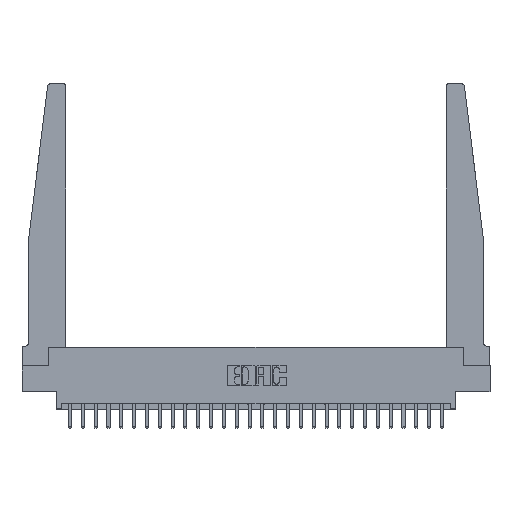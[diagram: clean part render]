
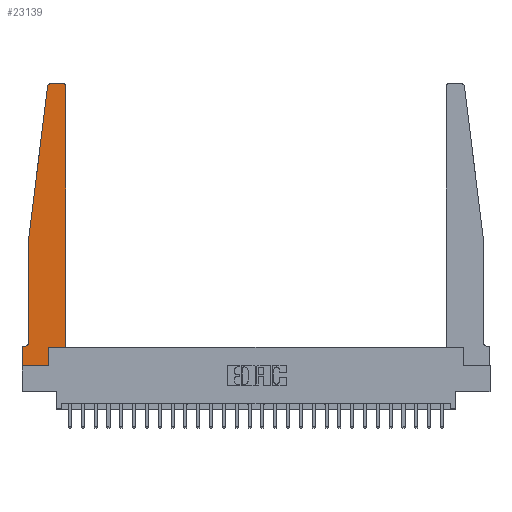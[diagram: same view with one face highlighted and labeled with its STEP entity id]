
A CAD part, top view. The second image highlights one B-rep face of the part: STEP entity #23139.
In plain terms, the highlighted planar face has unit normal (0, 0, 1).
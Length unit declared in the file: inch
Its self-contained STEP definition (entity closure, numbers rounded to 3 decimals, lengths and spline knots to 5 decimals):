
#36 = ORIENTED_EDGE ( 'NONE', *, *, #348, .T. ) ;
#49 = LINE ( 'NONE', #11934, #21082 ) ;
#164 = DIRECTION ( 'NONE',  ( -1., 0., 0. ) ) ;
#248 = CARTESIAN_POINT ( 'NONE',  ( 0., 0.1875, 0.37 ) ) ;
#348 = EDGE_CURVE ( 'NONE', #454, #18838, #3768, .T. ) ;
#454 = VERTEX_POINT ( 'NONE', #20134 ) ;
#847 = AXIS2_PLACEMENT_3D ( 'NONE', #1328, #15549, #3390 ) ;
#1015 = VECTOR ( 'NONE', #18648, 39.37008 ) ;
#1196 = CARTESIAN_POINT ( 'NONE',  ( 0.2605, 0.18, 0.37 ) ) ;
#1328 = CARTESIAN_POINT ( 'NONE',  ( 0.27653, 2.72, 0.37 ) ) ;
#1387 = CIRCLE ( 'NONE', #7462, 0.03 ) ;
#1421 = VECTOR ( 'NONE', #20547, 39.37008 ) ;
#1506 = DIRECTION ( 'NONE',  ( 1., 0., 0. ) ) ;
#1509 = DIRECTION ( 'NONE',  ( 0., 0., 1. ) ) ;
#1545 = CARTESIAN_POINT ( 'NONE',  ( 0.395, 2.72, 0.37 ) ) ;
#1833 = VECTOR ( 'NONE', #23311, 39.37008 ) ;
#2065 = ORIENTED_EDGE ( 'NONE', *, *, #13735, .T. ) ;
#2157 = VECTOR ( 'NONE', #19531, 39.37008 ) ;
#2487 = LINE ( 'NONE', #17197, #1833 ) ;
#2752 = ORIENTED_EDGE ( 'NONE', *, *, #12579, .T. ) ;
#2840 = ORIENTED_EDGE ( 'NONE', *, *, #25401, .T. ) ;
#3049 = LINE ( 'NONE', #17168, #24018 ) ;
#3324 = VERTEX_POINT ( 'NONE', #7595 ) ;
#3390 = DIRECTION ( 'NONE',  ( 1., 0., 0. ) ) ;
#3718 = EDGE_CURVE ( 'NONE', #18838, #4747, #1387, .T. ) ;
#3768 = LINE ( 'NONE', #21126, #24721 ) ;
#3822 = DIRECTION ( 'NONE',  ( 1., 0., 0. ) ) ;
#4447 = VERTEX_POINT ( 'NONE', #248 ) ;
#4747 = VERTEX_POINT ( 'NONE', #21454 ) ;
#5132 = CIRCLE ( 'NONE', #847, 0.03 ) ;
#5243 = DIRECTION ( 'NONE',  ( -1., 0., 0. ) ) ;
#5346 = CARTESIAN_POINT ( 'NONE',  ( 0.24675, 2.72367, 0.37 ) ) ;
#5848 = VECTOR ( 'NONE', #5243, 39.37008 ) ;
#6116 = CARTESIAN_POINT ( 'NONE',  ( 0., 0., 0.37 ) ) ;
#6149 = FACE_OUTER_BOUND ( 'NONE', #7897, .T. ) ;
#6227 = ORIENTED_EDGE ( 'NONE', *, *, #23930, .T. ) ;
#6298 = DIRECTION ( 'NONE',  ( 0., 0., 1. ) ) ;
#6418 = CARTESIAN_POINT ( 'NONE',  ( 0.065, 1.25, 0.37 ) ) ;
#6545 = CARTESIAN_POINT ( 'NONE',  ( 0., 0., 0.37 ) ) ;
#6699 = ORIENTED_EDGE ( 'NONE', *, *, #12045, .T. ) ;
#7462 = AXIS2_PLACEMENT_3D ( 'NONE', #1545, #1509, #1506 ) ;
#7467 = CARTESIAN_POINT ( 'NONE',  ( 0.065, 1.25, 0.37 ) ) ;
#7595 = CARTESIAN_POINT ( 'NONE',  ( 0.015, 0.1875, 0.37 ) ) ;
#7709 = VERTEX_POINT ( 'NONE', #1196 ) ;
#7897 = EDGE_LOOP ( 'NONE', ( #10655, #2065, #11889, #21381, #6227, #14574, #19105, #2752, #2840, #6699, #36, #18829 ) ) ;
#9648 = EDGE_CURVE ( 'NONE', #3324, #4447, #3049, .T. ) ;
#9666 = VECTOR ( 'NONE', #17566, 39.37008 ) ;
#9857 = VERTEX_POINT ( 'NONE', #22039 ) ;
#9939 = CIRCLE ( 'NONE', #15001, 0.05 ) ;
#10600 = AXIS2_PLACEMENT_3D ( 'NONE', #24430, #6298, #20430 ) ;
#10655 = ORIENTED_EDGE ( 'NONE', *, *, #20724, .T. ) ;
#11061 = VERTEX_POINT ( 'NONE', #6116 ) ;
#11240 = LINE ( 'NONE', #25395, #5848 ) ;
#11753 = CARTESIAN_POINT ( 'NONE',  ( 0.27653, 2.75, 0.37 ) ) ;
#11879 = LINE ( 'NONE', #6545, #1015 ) ;
#11889 = ORIENTED_EDGE ( 'NONE', *, *, #19004, .T. ) ;
#11891 = CARTESIAN_POINT ( 'NONE',  ( 0.425, 2.72, 0.37 ) ) ;
#11934 = CARTESIAN_POINT ( 'NONE',  ( 0.425, 0.18, 0.37 ) ) ;
#12045 = EDGE_CURVE ( 'NONE', #7709, #454, #49, .T. ) ;
#12270 = EDGE_CURVE ( 'NONE', #4447, #11061, #11879, .T. ) ;
#12363 = LINE ( 'NONE', #7467, #2157 ) ;
#12401 = DIRECTION ( 'NONE',  ( 0., 0., -1. ) ) ;
#12547 = VERTEX_POINT ( 'NONE', #5346 ) ;
#12579 = EDGE_CURVE ( 'NONE', #11061, #9857, #20389, .T. ) ;
#13735 = EDGE_CURVE ( 'NONE', #21817, #12547, #5132, .T. ) ;
#14574 = ORIENTED_EDGE ( 'NONE', *, *, #9648, .T. ) ;
#15001 = AXIS2_PLACEMENT_3D ( 'NONE', #24518, #12401, #164 ) ;
#15260 = VERTEX_POINT ( 'NONE', #18011 ) ;
#15503 = CARTESIAN_POINT ( 'NONE',  ( 0., 0., 0.37 ) ) ;
#15518 = VERTEX_POINT ( 'NONE', #23307 ) ;
#15549 = DIRECTION ( 'NONE',  ( 0., 0., 1. ) ) ;
#16383 = EDGE_CURVE ( 'NONE', #15260, #15518, #12363, .T. ) ;
#17168 = CARTESIAN_POINT ( 'NONE',  ( 0.065, 0.1875, 0.37 ) ) ;
#17197 = CARTESIAN_POINT ( 'NONE',  ( 0.2605, 0.18, 0.37 ) ) ;
#17566 = DIRECTION ( 'NONE',  ( 1., 0., 0. ) ) ;
#18011 = CARTESIAN_POINT ( 'NONE',  ( 0.065, 1.25, 0.37 ) ) ;
#18412 = PLANE ( 'NONE',  #10600 ) ;
#18648 = DIRECTION ( 'NONE',  ( 0., -1., 0. ) ) ;
#18829 = ORIENTED_EDGE ( 'NONE', *, *, #3718, .T. ) ;
#18838 = VERTEX_POINT ( 'NONE', #11891 ) ;
#19004 = EDGE_CURVE ( 'NONE', #12547, #15260, #22407, .T. ) ;
#19105 = ORIENTED_EDGE ( 'NONE', *, *, #12270, .T. ) ;
#19531 = DIRECTION ( 'NONE',  ( 0., -1., 0. ) ) ;
#20134 = CARTESIAN_POINT ( 'NONE',  ( 0.425, 0.18, 0.37 ) ) ;
#20389 = LINE ( 'NONE', #15503, #9666 ) ;
#20430 = DIRECTION ( 'NONE',  ( 1., 0., 0. ) ) ;
#20547 = DIRECTION ( 'NONE',  ( -0.122, -0.992, 0. ) ) ;
#20724 = EDGE_CURVE ( 'NONE', #4747, #21817, #11240, .T. ) ;
#21057 = DIRECTION ( 'NONE',  ( 0., 1., 0. ) ) ;
#21082 = VECTOR ( 'NONE', #3822, 39.37008 ) ;
#21126 = CARTESIAN_POINT ( 'NONE',  ( 0.425, 0.18, 0.37 ) ) ;
#21255 = DIRECTION ( 'NONE',  ( -1., 0., 0. ) ) ;
#21381 = ORIENTED_EDGE ( 'NONE', *, *, #16383, .T. ) ;
#21454 = CARTESIAN_POINT ( 'NONE',  ( 0.395, 2.75, 0.37 ) ) ;
#21817 = VERTEX_POINT ( 'NONE', #11753 ) ;
#22039 = CARTESIAN_POINT ( 'NONE',  ( 0.2605, 0., 0.37 ) ) ;
#22407 = LINE ( 'NONE', #6418, #1421 ) ;
#23139 = ADVANCED_FACE ( 'NONE', ( #6149 ), #18412, .T. ) ;
#23307 = CARTESIAN_POINT ( 'NONE',  ( 0.065, 0.2375, 0.37 ) ) ;
#23311 = DIRECTION ( 'NONE',  ( 0., 1., 0. ) ) ;
#23930 = EDGE_CURVE ( 'NONE', #15518, #3324, #9939, .T. ) ;
#24018 = VECTOR ( 'NONE', #21255, 39.37008 ) ;
#24430 = CARTESIAN_POINT ( 'NONE',  ( 0., 0.1875, 0.37 ) ) ;
#24518 = CARTESIAN_POINT ( 'NONE',  ( 0.015, 0.2375, 0.37 ) ) ;
#24721 = VECTOR ( 'NONE', #21057, 39.37008 ) ;
#25395 = CARTESIAN_POINT ( 'NONE',  ( 0.25, 2.75, 0.37 ) ) ;
#25401 = EDGE_CURVE ( 'NONE', #9857, #7709, #2487, .T. ) ;
